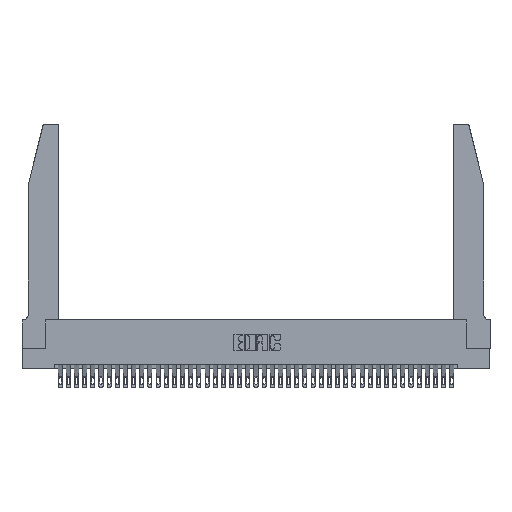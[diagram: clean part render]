
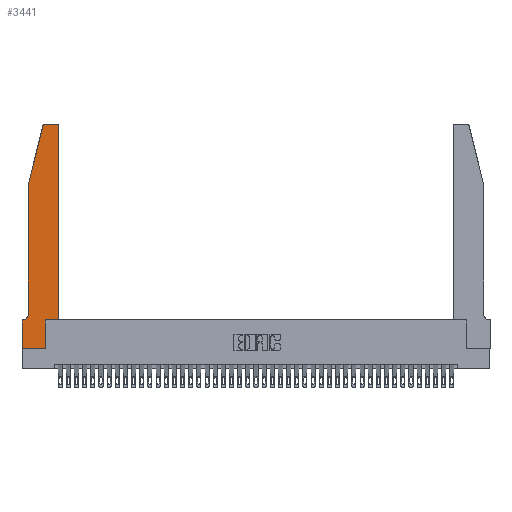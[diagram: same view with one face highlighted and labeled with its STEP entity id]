
A CAD part, top view. The second image highlights one B-rep face of the part: STEP entity #3441.
In plain terms, the highlighted planar face has unit normal (0, 0, 1).
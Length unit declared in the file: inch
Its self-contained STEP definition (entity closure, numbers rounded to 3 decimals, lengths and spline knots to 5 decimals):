
#18 = CARTESIAN_POINT ( 'NONE',  ( 0.0755, 0.35, 0.37 ) ) ;
#207 = ORIENTED_EDGE ( 'NONE', *, *, #12881, .T. ) ;
#999 = EDGE_CURVE ( 'NONE', #39594, #1653, #22526, .T. ) ;
#1646 = CARTESIAN_POINT ( 'NONE',  ( 0.2865, 0.35, 0.37 ) ) ;
#1653 = VERTEX_POINT ( 'NONE', #4856 ) ;
#1928 = LINE ( 'NONE', #28062, #11127 ) ;
#2494 = DIRECTION ( 'NONE',  ( 0., 0., 1. ) ) ;
#2604 = ORIENTED_EDGE ( 'NONE', *, *, #20621, .T. ) ;
#3441 = ADVANCED_FACE ( 'NONE', ( #9372 ), #21712, .T. ) ;
#3936 = LINE ( 'NONE', #25134, #36306 ) ;
#4295 = ORIENTED_EDGE ( 'NONE', *, *, #6632, .T. ) ;
#4852 = CARTESIAN_POINT ( 'NONE',  ( 0.4205, 2.72, 0.37 ) ) ;
#4856 = CARTESIAN_POINT ( 'NONE',  ( 0.0055, 0.35, 0.37 ) ) ;
#4988 = DIRECTION ( 'NONE',  ( 0., 0., 1. ) ) ;
#5069 = ORIENTED_EDGE ( 'NONE', *, *, #26423, .T. ) ;
#5597 = CARTESIAN_POINT ( 'NONE',  ( 0.4505, 0.35, 0.37 ) ) ;
#5626 = EDGE_CURVE ( 'NONE', #34469, #22605, #3936, .T. ) ;
#5846 = DIRECTION ( 'NONE',  ( 0., 0., -1. ) ) ;
#6233 = CARTESIAN_POINT ( 'NONE',  ( 0.284, 2.72, 0.37 ) ) ;
#6234 = CARTESIAN_POINT ( 'NONE',  ( 0.4505, 0.35, 0.37 ) ) ;
#6632 = EDGE_CURVE ( 'NONE', #15746, #25230, #23508, .T. ) ;
#6646 = VECTOR ( 'NONE', #29770, 39.37008 ) ;
#6799 = DIRECTION ( 'NONE',  ( -1., 0., 0. ) ) ;
#7088 = AXIS2_PLACEMENT_3D ( 'NONE', #25706, #5846, #15294 ) ;
#7572 = VECTOR ( 'NONE', #41915, 39.37008 ) ;
#8070 = EDGE_LOOP ( 'NONE', ( #12834, #5069, #32558, #207, #8215, #19179, #20404, #18367, #25272, #4295, #2604, #25567 ) ) ;
#8215 = ORIENTED_EDGE ( 'NONE', *, *, #999, .T. ) ;
#8717 = VECTOR ( 'NONE', #29327, 39.37008 ) ;
#9103 = VERTEX_POINT ( 'NONE', #27846 ) ;
#9372 = FACE_OUTER_BOUND ( 'NONE', #8070, .T. ) ;
#9457 = LINE ( 'NONE', #18, #25969 ) ;
#11127 = VECTOR ( 'NONE', #30129, 39.37008 ) ;
#11842 = EDGE_CURVE ( 'NONE', #36906, #26796, #35956, .T. ) ;
#12537 = CARTESIAN_POINT ( 'NONE',  ( 0.2865, 0.35, 0.37 ) ) ;
#12834 = ORIENTED_EDGE ( 'NONE', *, *, #5626, .T. ) ;
#12881 = EDGE_CURVE ( 'NONE', #26796, #39594, #1928, .T. ) ;
#12922 = AXIS2_PLACEMENT_3D ( 'NONE', #38357, #18650, #18068 ) ;
#14205 = VERTEX_POINT ( 'NONE', #20358 ) ;
#14222 = CARTESIAN_POINT ( 'NONE',  ( 0.0755, 2., 0.37 ) ) ;
#14296 = CARTESIAN_POINT ( 'NONE',  ( 0.2865, 0., 0.37 ) ) ;
#14943 = VECTOR ( 'NONE', #25397, 39.37008 ) ;
#15294 = DIRECTION ( 'NONE',  ( -1., 0., 0. ) ) ;
#15746 = VERTEX_POINT ( 'NONE', #1646 ) ;
#16338 = CARTESIAN_POINT ( 'NONE',  ( 0.4205, 2.75, 0.37 ) ) ;
#16834 = EDGE_CURVE ( 'NONE', #14205, #18999, #23722, .T. ) ;
#18068 = DIRECTION ( 'NONE',  ( 1., 0., 0. ) ) ;
#18238 = EDGE_CURVE ( 'NONE', #9103, #14205, #24140, .T. ) ;
#18367 = ORIENTED_EDGE ( 'NONE', *, *, #16834, .T. ) ;
#18650 = DIRECTION ( 'NONE',  ( 0., 0., 1. ) ) ;
#18999 = VERTEX_POINT ( 'NONE', #14296 ) ;
#19179 = ORIENTED_EDGE ( 'NONE', *, *, #37540, .T. ) ;
#19289 = CARTESIAN_POINT ( 'NONE',  ( 0.4505, 0.35, 0.37 ) ) ;
#20228 = CARTESIAN_POINT ( 'NONE',  ( 0.25487, 2.72718, 0.37 ) ) ;
#20358 = CARTESIAN_POINT ( 'NONE',  ( 0., 0., 0.37 ) ) ;
#20404 = ORIENTED_EDGE ( 'NONE', *, *, #18238, .T. ) ;
#20621 = EDGE_CURVE ( 'NONE', #25230, #21417, #40560, .T. ) ;
#20925 = AXIS2_PLACEMENT_3D ( 'NONE', #6233, #2494, #42334 ) ;
#21065 = CARTESIAN_POINT ( 'NONE',  ( 0., 0., 0.37 ) ) ;
#21417 = VERTEX_POINT ( 'NONE', #36318 ) ;
#21595 = DIRECTION ( 'NONE',  ( 0., 1., 0. ) ) ;
#21712 = PLANE ( 'NONE',  #12922 ) ;
#22526 = CIRCLE ( 'NONE', #7088, 0.07 ) ;
#22605 = VERTEX_POINT ( 'NONE', #29411 ) ;
#22611 = VECTOR ( 'NONE', #21595, 39.37008 ) ;
#23508 = LINE ( 'NONE', #6234, #7572 ) ;
#23722 = LINE ( 'NONE', #41763, #14943 ) ;
#24140 = LINE ( 'NONE', #21065, #6646 ) ;
#24544 = CARTESIAN_POINT ( 'NONE',  ( 0.0755, 0.42, 0.37 ) ) ;
#24597 = EDGE_CURVE ( 'NONE', #18999, #15746, #42183, .T. ) ;
#25134 = CARTESIAN_POINT ( 'NONE',  ( 0.2605, 2.75, 0.37 ) ) ;
#25230 = VERTEX_POINT ( 'NONE', #19289 ) ;
#25272 = ORIENTED_EDGE ( 'NONE', *, *, #24597, .T. ) ;
#25284 = DIRECTION ( 'NONE',  ( -1., 0., 0. ) ) ;
#25397 = DIRECTION ( 'NONE',  ( 1., 0., 0. ) ) ;
#25567 = ORIENTED_EDGE ( 'NONE', *, *, #31221, .T. ) ;
#25706 = CARTESIAN_POINT ( 'NONE',  ( 0.0055, 0.42, 0.37 ) ) ;
#25969 = VECTOR ( 'NONE', #6799, 39.37008 ) ;
#26094 = CIRCLE ( 'NONE', #26526, 0.03 ) ;
#26423 = EDGE_CURVE ( 'NONE', #22605, #36906, #40778, .T. ) ;
#26526 = AXIS2_PLACEMENT_3D ( 'NONE', #4852, #4988, #31141 ) ;
#26796 = VERTEX_POINT ( 'NONE', #14222 ) ;
#27846 = CARTESIAN_POINT ( 'NONE',  ( 0., 0.35, 0.37 ) ) ;
#28062 = CARTESIAN_POINT ( 'NONE',  ( 0.0755, 2., 0.37 ) ) ;
#29327 = DIRECTION ( 'NONE',  ( -0.239, -0.971, 0. ) ) ;
#29411 = CARTESIAN_POINT ( 'NONE',  ( 0.284, 2.75, 0.37 ) ) ;
#29770 = DIRECTION ( 'NONE',  ( 0., -1., 0. ) ) ;
#30129 = DIRECTION ( 'NONE',  ( 0., -1., 0. ) ) ;
#31141 = DIRECTION ( 'NONE',  ( 1., 0., 0. ) ) ;
#31221 = EDGE_CURVE ( 'NONE', #21417, #34469, #26094, .T. ) ;
#32558 = ORIENTED_EDGE ( 'NONE', *, *, #11842, .T. ) ;
#33356 = VECTOR ( 'NONE', #35133, 39.37008 ) ;
#34469 = VERTEX_POINT ( 'NONE', #16338 ) ;
#35133 = DIRECTION ( 'NONE',  ( 0., 1., 0. ) ) ;
#35766 = CARTESIAN_POINT ( 'NONE',  ( 0.0755, 2., 0.37 ) ) ;
#35956 = LINE ( 'NONE', #35766, #8717 ) ;
#36306 = VECTOR ( 'NONE', #25284, 39.37008 ) ;
#36318 = CARTESIAN_POINT ( 'NONE',  ( 0.4505, 2.72, 0.37 ) ) ;
#36906 = VERTEX_POINT ( 'NONE', #20228 ) ;
#37540 = EDGE_CURVE ( 'NONE', #1653, #9103, #9457, .T. ) ;
#38357 = CARTESIAN_POINT ( 'NONE',  ( 0., 0.35, 0.37 ) ) ;
#39594 = VERTEX_POINT ( 'NONE', #24544 ) ;
#40560 = LINE ( 'NONE', #5597, #22611 ) ;
#40778 = CIRCLE ( 'NONE', #20925, 0.03 ) ;
#41763 = CARTESIAN_POINT ( 'NONE',  ( 0., 0., 0.37 ) ) ;
#41915 = DIRECTION ( 'NONE',  ( 1., 0., 0. ) ) ;
#42183 = LINE ( 'NONE', #12537, #33356 ) ;
#42334 = DIRECTION ( 'NONE',  ( 1., 0., 0. ) ) ;
